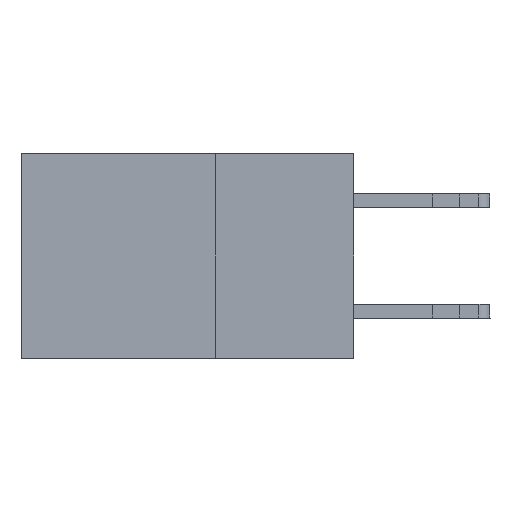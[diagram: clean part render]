
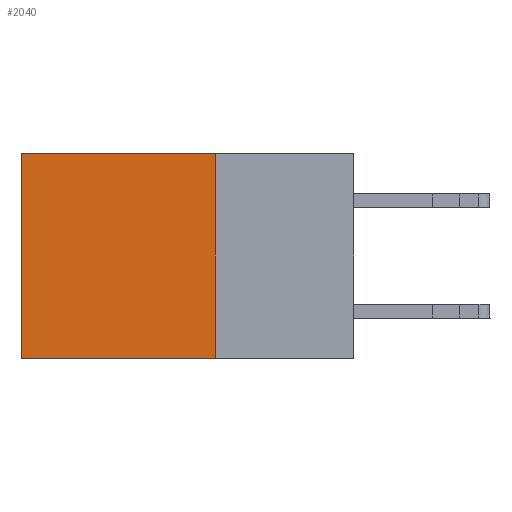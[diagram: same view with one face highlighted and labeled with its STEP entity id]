
A CAD part, left-side view. The second image highlights one B-rep face of the part: STEP entity #2040.
In plain terms, the highlighted planar face has unit normal (-1, 0, 0).
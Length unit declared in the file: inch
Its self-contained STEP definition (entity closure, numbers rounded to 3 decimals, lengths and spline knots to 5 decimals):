
#1205 = VERTEX_POINT ( 'NONE', #14458 ) ;
#1675 = CARTESIAN_POINT ( 'NONE',  ( 0.2875, 0.6, 0. ) ) ;
#2032 = LINE ( 'NONE', #15393, #2693 ) ;
#2040 = ADVANCED_FACE ( 'NONE', ( #6491 ), #18946, .F. ) ;
#2693 = VECTOR ( 'NONE', #8929, 39.37008 ) ;
#2816 = VERTEX_POINT ( 'NONE', #9148 ) ;
#3442 = DIRECTION ( 'NONE',  ( 0., 0., -1. ) ) ;
#4172 = CARTESIAN_POINT ( 'NONE',  ( 0.2875, 0.25, 0. ) ) ;
#4411 = LINE ( 'NONE', #21085, #5067 ) ;
#5067 = VECTOR ( 'NONE', #19128, 39.37008 ) ;
#6253 = CARTESIAN_POINT ( 'NONE',  ( 0.2875, 0.25, 0. ) ) ;
#6491 = FACE_OUTER_BOUND ( 'NONE', #12541, .T. ) ;
#7743 = VECTOR ( 'NONE', #21271, 39.37008 ) ;
#8387 = DIRECTION ( 'NONE',  ( 1., 0., 0. ) ) ;
#8633 = VERTEX_POINT ( 'NONE', #23819 ) ;
#8929 = DIRECTION ( 'NONE',  ( 0., 1., 0. ) ) ;
#9148 = CARTESIAN_POINT ( 'NONE',  ( 0.2875, 0.25, -0.37 ) ) ;
#9233 = ORIENTED_EDGE ( 'NONE', *, *, #20122, .F. ) ;
#11163 = EDGE_CURVE ( 'NONE', #2816, #8633, #2032, .T. ) ;
#11356 = VERTEX_POINT ( 'NONE', #11490 ) ;
#11490 = CARTESIAN_POINT ( 'NONE',  ( 0.2875, 0.6, 0. ) ) ;
#12443 = DIRECTION ( 'NONE',  ( 0., 0., -1. ) ) ;
#12541 = EDGE_LOOP ( 'NONE', ( #14240, #14225, #9233, #20873 ) ) ;
#14225 = ORIENTED_EDGE ( 'NONE', *, *, #11163, .F. ) ;
#14240 = ORIENTED_EDGE ( 'NONE', *, *, #27396, .T. ) ;
#14458 = CARTESIAN_POINT ( 'NONE',  ( 0.2875, 0.25, 0. ) ) ;
#14830 = LINE ( 'NONE', #1675, #26181 ) ;
#15393 = CARTESIAN_POINT ( 'NONE',  ( 0.2875, 0.25, -0.37 ) ) ;
#16886 = AXIS2_PLACEMENT_3D ( 'NONE', #6253, #8387, #3442 ) ;
#18341 = LINE ( 'NONE', #4172, #7743 ) ;
#18946 = PLANE ( 'NONE',  #16886 ) ;
#19128 = DIRECTION ( 'NONE',  ( 0., 1., 0. ) ) ;
#20122 = EDGE_CURVE ( 'NONE', #1205, #2816, #18341, .T. ) ;
#20127 = EDGE_CURVE ( 'NONE', #1205, #11356, #4411, .T. ) ;
#20873 = ORIENTED_EDGE ( 'NONE', *, *, #20127, .T. ) ;
#21085 = CARTESIAN_POINT ( 'NONE',  ( 0.2875, 0.25, 0. ) ) ;
#21271 = DIRECTION ( 'NONE',  ( 0., 0., -1. ) ) ;
#23819 = CARTESIAN_POINT ( 'NONE',  ( 0.2875, 0.6, -0.37 ) ) ;
#26181 = VECTOR ( 'NONE', #12443, 39.37008 ) ;
#27396 = EDGE_CURVE ( 'NONE', #11356, #8633, #14830, .T. ) ;
